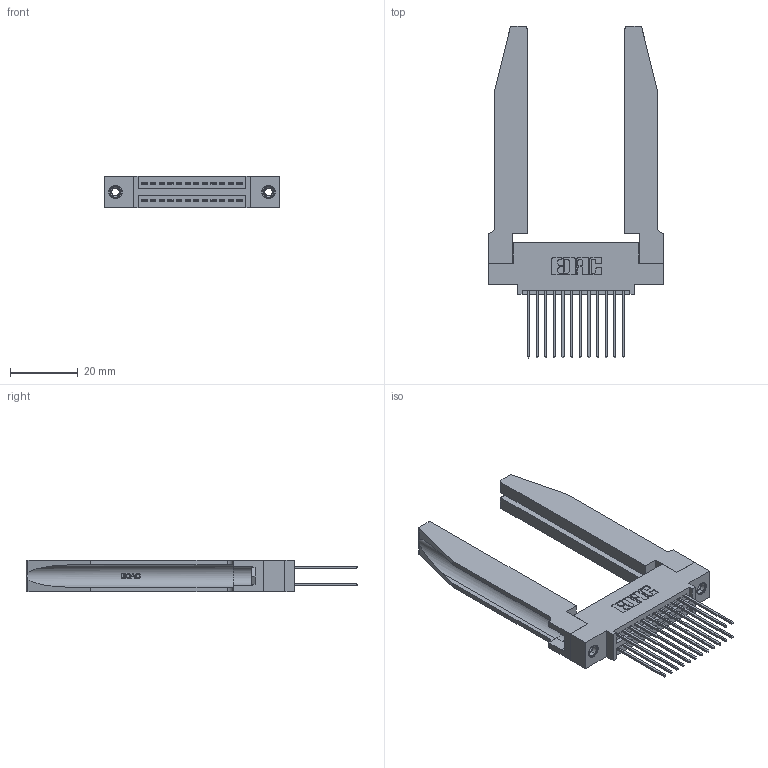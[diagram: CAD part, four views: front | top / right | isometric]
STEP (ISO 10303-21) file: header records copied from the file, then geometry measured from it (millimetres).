
FILE_DESCRIPTION (( 'STEP AP203' ), '1' );
FILE_NAME ('345-024-541-578.STEP', '2019-10-27T17:06:42', ( '' ), ( '' ), 'SwSTEP 2.0', 'SolidWorks 2016', '' );
FILE_SCHEMA (( 'CONFIG_CONTROL_DESIGN' ));
Length unit declared in the file: inch
Products named in the file (5): 345-250-001_345-250-001-102; 345-220-078_345-220-078; 345-292-001_345-293-141; 345-024-541-578; 345 Part_0.110 Offset - 0.156 Dia-TH
Assembly tree (29 placements, depth 2):
  345-024-541-578
    345 Part_0.110 Offset - 0.156 Dia-TH
    345-292-001_345-293-141  x24
    345-250-001_345-250-001-102  x2
    345-220-078_345-220-078  x2
Bounding box: 51.71 x 97.71 x 9.4 mm (x, y, z)
Volume: 12579.9 mm3; surface area: 14106.7 mm2
Topology: 29 solids, 29 shells, 1564 faces, 4537 edges, 2982 vertices
Faces by surface type: plane 1018, cylinder 494, bspline 36, cone 12, torus 4
Entity records: 18344 total; most frequent: CARTESIAN_POINT 4023, ORIENTED_EDGE 2854, DIRECTION 2577, EDGE_CURVE 1427, VECTOR 1153, LINE 1153, VERTEX_POINT 944, AXIS2_PLACEMENT_3D 712
